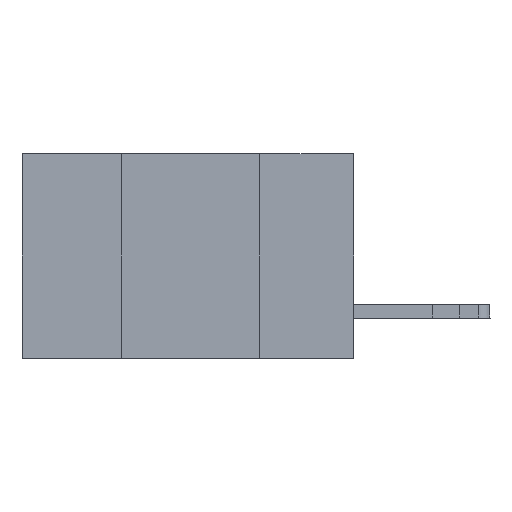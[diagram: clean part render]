
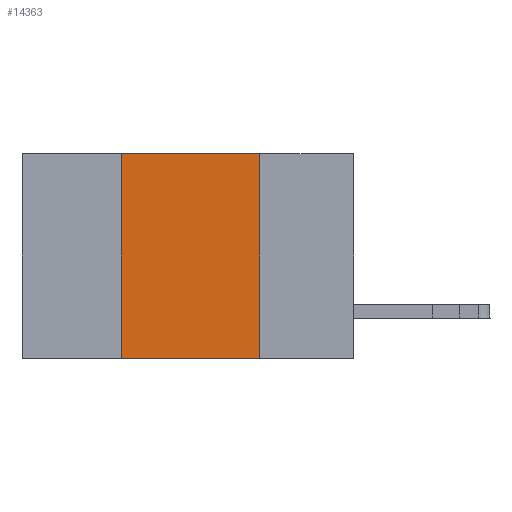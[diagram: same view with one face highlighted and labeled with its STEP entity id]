
A CAD part, left-side view. The second image highlights one B-rep face of the part: STEP entity #14363.
In plain terms, the highlighted planar face has unit normal (-1, 0, 0).
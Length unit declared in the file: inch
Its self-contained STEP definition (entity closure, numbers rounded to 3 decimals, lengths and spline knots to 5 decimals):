
#465 = VECTOR ( 'NONE', #11806, 39.37008 ) ;
#2095 = LINE ( 'NONE', #5367, #7365 ) ;
#3110 = CARTESIAN_POINT ( 'NONE',  ( 0., 0.6, 0. ) ) ;
#4000 = CARTESIAN_POINT ( 'NONE',  ( 0., 0.42, -0.37 ) ) ;
#5367 = CARTESIAN_POINT ( 'NONE',  ( 0., 0.17, 0. ) ) ;
#6721 = CARTESIAN_POINT ( 'NONE',  ( 0., 0.6, 0. ) ) ;
#7365 = VECTOR ( 'NONE', #26843, 39.37008 ) ;
#9108 = AXIS2_PLACEMENT_3D ( 'NONE', #3110, #25316, #13857 ) ;
#10044 = CARTESIAN_POINT ( 'NONE',  ( 0., 0.17, -0.37 ) ) ;
#10159 = VERTEX_POINT ( 'NONE', #10044 ) ;
#10251 = LINE ( 'NONE', #15156, #11008 ) ;
#11008 = VECTOR ( 'NONE', #23895, 39.37008 ) ;
#11806 = DIRECTION ( 'NONE',  ( 0., -1., 0. ) ) ;
#13857 = DIRECTION ( 'NONE',  ( 0., 0., -1. ) ) ;
#14363 = ADVANCED_FACE ( 'NONE', ( #22562 ), #24783, .F. ) ;
#15156 = CARTESIAN_POINT ( 'NONE',  ( 0., 0.42, 0. ) ) ;
#15545 = VECTOR ( 'NONE', #17519, 39.37008 ) ;
#16097 = ORIENTED_EDGE ( 'NONE', *, *, #22317, .T. ) ;
#16489 = ORIENTED_EDGE ( 'NONE', *, *, #27498, .F. ) ;
#17161 = LINE ( 'NONE', #19547, #15545 ) ;
#17519 = DIRECTION ( 'NONE',  ( 0., -1., 0. ) ) ;
#17603 = CARTESIAN_POINT ( 'NONE',  ( 0., 0.17, 0. ) ) ;
#17946 = ORIENTED_EDGE ( 'NONE', *, *, #21455, .F. ) ;
#19547 = CARTESIAN_POINT ( 'NONE',  ( 0., 0.6, -0.37 ) ) ;
#21455 = EDGE_CURVE ( 'NONE', #28479, #27964, #28726, .T. ) ;
#21917 = EDGE_LOOP ( 'NONE', ( #16489, #17946, #24228, #16097 ) ) ;
#22317 = EDGE_CURVE ( 'NONE', #34446, #10159, #17161, .T. ) ;
#22562 = FACE_OUTER_BOUND ( 'NONE', #21917, .T. ) ;
#23895 = DIRECTION ( 'NONE',  ( 0., 0., 1. ) ) ;
#24228 = ORIENTED_EDGE ( 'NONE', *, *, #31275, .F. ) ;
#24783 = PLANE ( 'NONE',  #9108 ) ;
#25316 = DIRECTION ( 'NONE',  ( 1., 0., 0. ) ) ;
#26843 = DIRECTION ( 'NONE',  ( 0., 0., -1. ) ) ;
#27498 = EDGE_CURVE ( 'NONE', #27964, #10159, #2095, .T. ) ;
#27795 = CARTESIAN_POINT ( 'NONE',  ( 0., 0.42, 0. ) ) ;
#27964 = VERTEX_POINT ( 'NONE', #17603 ) ;
#28479 = VERTEX_POINT ( 'NONE', #27795 ) ;
#28726 = LINE ( 'NONE', #6721, #465 ) ;
#31275 = EDGE_CURVE ( 'NONE', #34446, #28479, #10251, .T. ) ;
#34446 = VERTEX_POINT ( 'NONE', #4000 ) ;
